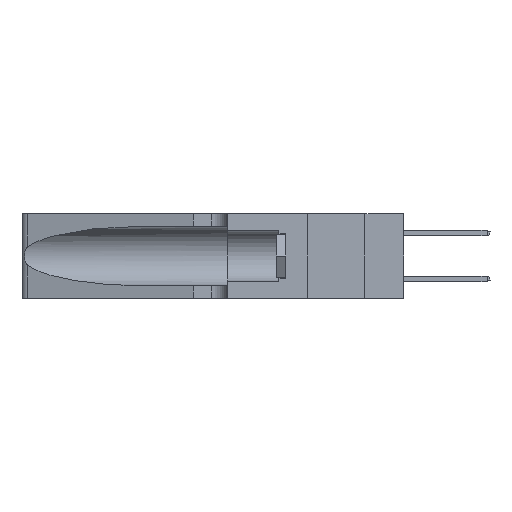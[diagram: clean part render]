
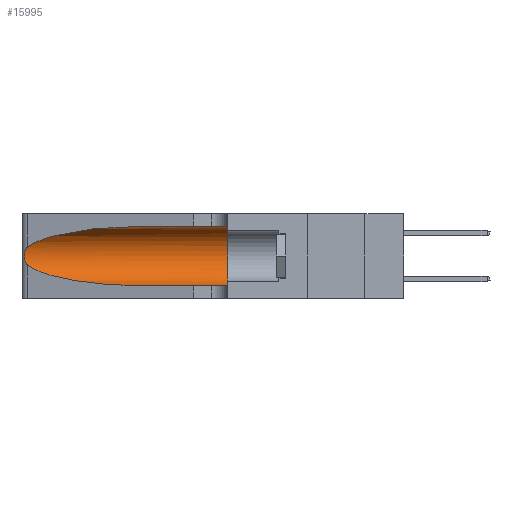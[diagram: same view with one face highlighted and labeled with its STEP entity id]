
A CAD part, left-side view. The second image highlights one B-rep face of the part: STEP entity #15995.
In plain terms, the highlighted cylindrical face has radius 3.308 mm (diameter 6.617 mm), a partial arc.
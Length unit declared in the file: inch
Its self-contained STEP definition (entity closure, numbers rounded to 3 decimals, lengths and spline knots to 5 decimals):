
#605 = ORIENTED_EDGE ( 'NONE', *, *, #15537, .F. ) ;
#980 = CARTESIAN_POINT ( 'NONE',  ( 0.2373, 1.15595, 0.28018 ) ) ;
#1335 = ORIENTED_EDGE ( 'NONE', *, *, #27975, .F. ) ;
#1613 = VERTEX_POINT ( 'NONE', #25091 ) ;
#2215 = CARTESIAN_POINT ( 'NONE',  ( 0.26018, 1.23835, 0.19895 ) ) ;
#2251 = LINE ( 'NONE', #5156, #7895 ) ;
#3081 = AXIS2_PLACEMENT_3D ( 'NONE', #3543, #19881, #5994 ) ;
#3459 = CARTESIAN_POINT ( 'NONE',  ( 0.25487, 1.22718, 0.22369 ) ) ;
#3543 = CARTESIAN_POINT ( 'NONE',  ( 0.1305, 0.35, 0.185 ) ) ;
#4646 = CARTESIAN_POINT ( 'NONE',  ( 0.26075, 1.23896, 0.178 ) ) ;
#5156 = CARTESIAN_POINT ( 'NONE',  ( 0.1305, 1.61858, 0.31525 ) ) ;
#5638 = EDGE_CURVE ( 'NONE', #13425, #19745, #26851, .T. ) ;
#5986 = CARTESIAN_POINT ( 'NONE',  ( 0.18966, 0.96281, 0.05475 ) ) ;
#5994 = DIRECTION ( 'NONE',  ( 0., 0., 1. ) ) ;
#7074 = CARTESIAN_POINT ( 'NONE',  ( 0.25856, 1.23593, 0.16098 ) ) ;
#7555 = DIRECTION ( 'NONE',  ( 0., -1., 0. ) ) ;
#7589 = CIRCLE ( 'NONE', #3081, 0.13025 ) ;
#7895 = VECTOR ( 'NONE', #23677, 39.37008 ) ;
#9316 = CARTESIAN_POINT ( 'NONE',  ( 0.25487, 1.22718, 0.22369 ) ) ;
#9361 =( BOUNDED_CURVE ( )  B_SPLINE_CURVE ( 3, ( #28838, #21958, #980, #17424 ),
 .UNSPECIFIED., .F., .F. ) 
 B_SPLINE_CURVE_WITH_KNOTS ( ( 4, 4 ),
 ( 1.5708, 2.84003 ),
 .UNSPECIFIED. ) 
 CURVE ( )  GEOMETRIC_REPRESENTATION_ITEM ( )  RATIONAL_B_SPLINE_CURVE ( ( 1., 0.87, 0.87, 1. ) ) 
 REPRESENTATION_ITEM ( '' )  );
#9418 = CARTESIAN_POINT ( 'NONE',  ( 0.25639, 1.23186, 0.15144 ) ) ;
#9738 = CARTESIAN_POINT ( 'NONE',  ( 0.1305, 1.61858, 0.185 ) ) ;
#10223 = CARTESIAN_POINT ( 'NONE',  ( 0.1305, 0.35, 0.05475 ) ) ;
#10816 = CARTESIAN_POINT ( 'NONE',  ( 0.1305, 0.35, 0.31525 ) ) ;
#10976 = ORIENTED_EDGE ( 'NONE', *, *, #22801, .T. ) ;
#11763 = CARTESIAN_POINT ( 'NONE',  ( 0.25487, 1.22718, 0.14631 ) ) ;
#12002 = AXIS2_PLACEMENT_3D ( 'NONE', #9738, #25894, #12084 ) ;
#12084 = DIRECTION ( 'NONE',  ( 0., 0., -1. ) ) ;
#13425 = VERTEX_POINT ( 'NONE', #23197 ) ;
#13749 = VERTEX_POINT ( 'NONE', #3459 ) ;
#14012 = CARTESIAN_POINT ( 'NONE',  ( 0.25639, 1.23184, 0.21858 ) ) ;
#15537 = EDGE_CURVE ( 'NONE', #19124, #25841, #7589, .T. ) ;
#15995 = ADVANCED_FACE ( 'NONE', ( #18452 ), #23814, .F. ) ;
#16342 = CARTESIAN_POINT ( 'NONE',  ( 0.25854, 1.2359, 0.20912 ) ) ;
#16657 = EDGE_CURVE ( 'NONE', #19745, #25841, #23405, .T. ) ;
#16805 = CARTESIAN_POINT ( 'NONE',  ( 0.1305, 1.61858, 0.05475 ) ) ;
#17338 = VECTOR ( 'NONE', #7555, 39.37008 ) ;
#17424 = CARTESIAN_POINT ( 'NONE',  ( 0.25487, 1.22718, 0.22369 ) ) ;
#18452 = FACE_OUTER_BOUND ( 'NONE', #20701, .T. ) ;
#18576 = ORIENTED_EDGE ( 'NONE', *, *, #16657, .T. ) ;
#18617 = CARTESIAN_POINT ( 'NONE',  ( 0.26075, 1.23896, 0.19203 ) ) ;
#19124 = VERTEX_POINT ( 'NONE', #10816 ) ;
#19745 = VERTEX_POINT ( 'NONE', #26710 ) ;
#19881 = DIRECTION ( 'NONE',  ( 0., 1., 0. ) ) ;
#20590 = B_SPLINE_CURVE_WITH_KNOTS ( 'NONE', 3,
 ( #9316, #29940, #14012, #30028, #16342, #2215, #18617, #4646, #20946, #7074, #23218, #9418, #25557, #11763 ),
 .UNSPECIFIED., .F., .F.,
 ( 4, 2, 2, 2, 2, 2, 4 ),
 ( 0., 0.00027, 0.00053, 0.00107, 0.0016, 0.00187, 0.00214 ),
 .UNSPECIFIED. ) ;
#20701 = EDGE_LOOP ( 'NONE', ( #22542, #10976, #30036, #18576, #605, #1335 ) ) ;
#20946 = CARTESIAN_POINT ( 'NONE',  ( 0.26017, 1.23833, 0.17102 ) ) ;
#21958 = CARTESIAN_POINT ( 'NONE',  ( 0.18966, 0.96281, 0.31525 ) ) ;
#22187 = CARTESIAN_POINT ( 'NONE',  ( 0.2373, 1.15595, 0.08982 ) ) ;
#22542 = ORIENTED_EDGE ( 'NONE', *, *, #27485, .T. ) ;
#22801 = EDGE_CURVE ( 'NONE', #13749, #13425, #20590, .T. ) ;
#23197 = CARTESIAN_POINT ( 'NONE',  ( 0.25487, 1.22718, 0.14631 ) ) ;
#23218 = CARTESIAN_POINT ( 'NONE',  ( 0.25789, 1.23486, 0.15765 ) ) ;
#23405 = LINE ( 'NONE', #16805, #17338 ) ;
#23677 = DIRECTION ( 'NONE',  ( 0., -1., 0. ) ) ;
#23814 = CYLINDRICAL_SURFACE ( 'NONE', #12002, 0.13025 ) ;
#24476 = CARTESIAN_POINT ( 'NONE',  ( 0.1305, 0.72297, 0.05475 ) ) ;
#25091 = CARTESIAN_POINT ( 'NONE',  ( 0.1305, 0.72297, 0.31525 ) ) ;
#25557 = CARTESIAN_POINT ( 'NONE',  ( 0.25555, 1.22993, 0.14849 ) ) ;
#25841 = VERTEX_POINT ( 'NONE', #10223 ) ;
#25894 = DIRECTION ( 'NONE',  ( 0., -1., 0. ) ) ;
#26710 = CARTESIAN_POINT ( 'NONE',  ( 0.1305, 0.72297, 0.05475 ) ) ;
#26714 = CARTESIAN_POINT ( 'NONE',  ( 0.25487, 1.22718, 0.14631 ) ) ;
#26851 =( BOUNDED_CURVE ( )  B_SPLINE_CURVE ( 3, ( #26714, #22187, #5986, #24476 ),
 .UNSPECIFIED., .F., .T. ) 
 B_SPLINE_CURVE_WITH_KNOTS ( ( 4, 4 ),
 ( 3.44316, 4.71239 ),
 .UNSPECIFIED. ) 
 CURVE ( )  GEOMETRIC_REPRESENTATION_ITEM ( )  RATIONAL_B_SPLINE_CURVE ( ( 1., 0.87, 0.87, 1. ) ) 
 REPRESENTATION_ITEM ( '' )  );
#27485 = EDGE_CURVE ( 'NONE', #1613, #13749, #9361, .T. ) ;
#27975 = EDGE_CURVE ( 'NONE', #1613, #19124, #2251, .T. ) ;
#28838 = CARTESIAN_POINT ( 'NONE',  ( 0.1305, 0.72297, 0.31525 ) ) ;
#29940 = CARTESIAN_POINT ( 'NONE',  ( 0.25555, 1.22994, 0.2215 ) ) ;
#30028 = CARTESIAN_POINT ( 'NONE',  ( 0.25787, 1.23484, 0.2124 ) ) ;
#30036 = ORIENTED_EDGE ( 'NONE', *, *, #5638, .T. ) ;
